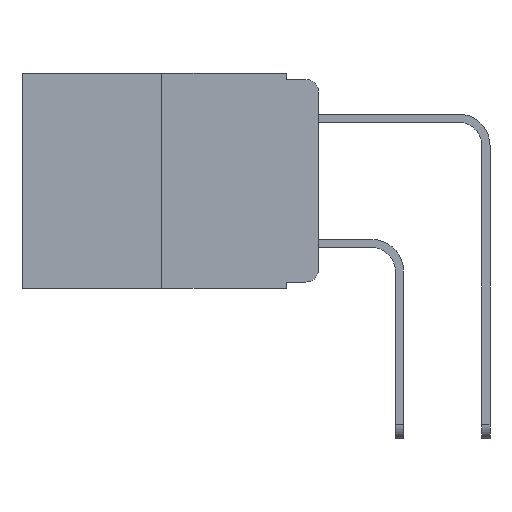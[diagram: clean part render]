
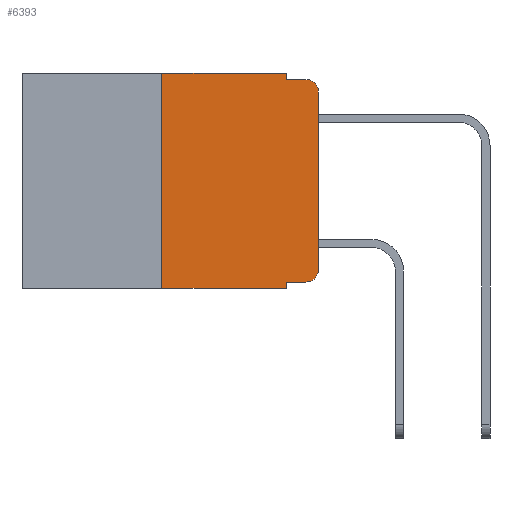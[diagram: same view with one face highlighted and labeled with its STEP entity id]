
A CAD part, left-side view. The second image highlights one B-rep face of the part: STEP entity #6393.
In plain terms, the highlighted planar face has unit normal (-1, 0, 0).
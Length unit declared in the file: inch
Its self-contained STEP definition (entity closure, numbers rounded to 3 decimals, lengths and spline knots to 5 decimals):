
#328 = ORIENTED_EDGE ( 'NONE', *, *, #4727, .F. ) ;
#359 = CIRCLE ( 'NONE', #1858, 0.02 ) ;
#385 = DIRECTION ( 'NONE',  ( -1., 0., 0. ) ) ;
#634 = ORIENTED_EDGE ( 'NONE', *, *, #3412, .T. ) ;
#791 = ORIENTED_EDGE ( 'NONE', *, *, #3538, .F. ) ;
#983 = VECTOR ( 'NONE', #6883, 39.37008 ) ;
#1095 = ORIENTED_EDGE ( 'NONE', *, *, #1416, .T. ) ;
#1416 = EDGE_CURVE ( 'NONE', #10333, #5225, #6491, .T. ) ;
#1601 = VECTOR ( 'NONE', #13738, 39.37008 ) ;
#1858 = AXIS2_PLACEMENT_3D ( 'NONE', #7493, #385, #8627 ) ;
#2063 = CARTESIAN_POINT ( 'NONE',  ( 0., 0.473, 0. ) ) ;
#2065 = PLANE ( 'NONE',  #14643 ) ;
#2159 = CIRCLE ( 'NONE', #10246, 0.02 ) ;
#2265 = ORIENTED_EDGE ( 'NONE', *, *, #6985, .T. ) ;
#2274 = EDGE_CURVE ( 'NONE', #12450, #3481, #10789, .T. ) ;
#2370 = CARTESIAN_POINT ( 'NONE',  ( 0., 0., -0.313 ) ) ;
#2591 = CARTESIAN_POINT ( 'NONE',  ( 0., 0.051, -0.333 ) ) ;
#2628 = ORIENTED_EDGE ( 'NONE', *, *, #2274, .F. ) ;
#2881 = CARTESIAN_POINT ( 'NONE',  ( 0., 0., 0. ) ) ;
#3010 = VECTOR ( 'NONE', #8505, 39.37008 ) ;
#3142 = VECTOR ( 'NONE', #12674, 39.37008 ) ;
#3370 = VERTEX_POINT ( 'NONE', #8922 ) ;
#3405 = DIRECTION ( 'NONE',  ( 0., 0., -1. ) ) ;
#3412 = EDGE_CURVE ( 'NONE', #5357, #10333, #2159, .T. ) ;
#3481 = VERTEX_POINT ( 'NONE', #6370 ) ;
#3538 = EDGE_CURVE ( 'NONE', #3481, #3671, #9909, .T. ) ;
#3671 = VERTEX_POINT ( 'NONE', #13999 ) ;
#3916 = EDGE_CURVE ( 'NONE', #3671, #13703, #9902, .T. ) ;
#4099 = DIRECTION ( 'NONE',  ( 0., -1., 0. ) ) ;
#4421 = EDGE_LOOP ( 'NONE', ( #1095, #2265, #328, #5591, #791, #2628, #11192, #5495, #7170, #634 ) ) ;
#4689 = DIRECTION ( 'NONE',  ( 0., 0., -1. ) ) ;
#4707 = DIRECTION ( 'NONE',  ( 1., 0., 0. ) ) ;
#4727 = EDGE_CURVE ( 'NONE', #13703, #3370, #6270, .T. ) ;
#4757 = VERTEX_POINT ( 'NONE', #12067 ) ;
#5158 = VECTOR ( 'NONE', #4099, 39.37008 ) ;
#5159 = CARTESIAN_POINT ( 'NONE',  ( 0., 0.473, 0. ) ) ;
#5225 = VERTEX_POINT ( 'NONE', #14273 ) ;
#5357 = VERTEX_POINT ( 'NONE', #7794 ) ;
#5495 = ORIENTED_EDGE ( 'NONE', *, *, #7742, .F. ) ;
#5583 = LINE ( 'NONE', #2591, #13869 ) ;
#5591 = ORIENTED_EDGE ( 'NONE', *, *, #3916, .F. ) ;
#6252 = DIRECTION ( 'NONE',  ( 0., 0., -1. ) ) ;
#6270 = LINE ( 'NONE', #11668, #3142 ) ;
#6271 = DIRECTION ( 'NONE',  ( 0., -1., 0. ) ) ;
#6336 = EDGE_CURVE ( 'NONE', #12450, #4757, #8492, .T. ) ;
#6370 = CARTESIAN_POINT ( 'NONE',  ( 0., 0.25, 0. ) ) ;
#6393 = ADVANCED_FACE ( 'NONE', ( #13505 ), #2065, .F. ) ;
#6491 = LINE ( 'NONE', #2881, #3010 ) ;
#6554 = CARTESIAN_POINT ( 'NONE',  ( 0., 0.25, -0.343 ) ) ;
#6874 = CARTESIAN_POINT ( 'NONE',  ( 0., 0.051, -0.333 ) ) ;
#6883 = DIRECTION ( 'NONE',  ( 0., 0., -1. ) ) ;
#6985 = EDGE_CURVE ( 'NONE', #5225, #3370, #359, .T. ) ;
#7009 = CARTESIAN_POINT ( 'NONE',  ( 0., 0.051, 0. ) ) ;
#7170 = ORIENTED_EDGE ( 'NONE', *, *, #9983, .T. ) ;
#7493 = CARTESIAN_POINT ( 'NONE',  ( 0., 0.02, -0.03 ) ) ;
#7742 = EDGE_CURVE ( 'NONE', #10996, #4757, #10012, .T. ) ;
#7794 = CARTESIAN_POINT ( 'NONE',  ( 0., 0.02, -0.333 ) ) ;
#8417 = DIRECTION ( 'NONE',  ( 0., -1., 0. ) ) ;
#8492 = LINE ( 'NONE', #13337, #5158 ) ;
#8505 = DIRECTION ( 'NONE',  ( 0., 0., 1. ) ) ;
#8627 = DIRECTION ( 'NONE',  ( 0., 0., -1. ) ) ;
#8922 = CARTESIAN_POINT ( 'NONE',  ( 0., 0.02, -0.01 ) ) ;
#9902 = LINE ( 'NONE', #7009, #983 ) ;
#9909 = LINE ( 'NONE', #5159, #12722 ) ;
#9983 = EDGE_CURVE ( 'NONE', #10996, #5357, #5583, .T. ) ;
#10012 = LINE ( 'NONE', #14340, #13465 ) ;
#10246 = AXIS2_PLACEMENT_3D ( 'NONE', #11680, #10644, #6252 ) ;
#10333 = VERTEX_POINT ( 'NONE', #2370 ) ;
#10466 = CARTESIAN_POINT ( 'NONE',  ( 0., 0.25, 0. ) ) ;
#10644 = DIRECTION ( 'NONE',  ( -1., 0., 0. ) ) ;
#10789 = LINE ( 'NONE', #10466, #1601 ) ;
#10996 = VERTEX_POINT ( 'NONE', #6874 ) ;
#11192 = ORIENTED_EDGE ( 'NONE', *, *, #6336, .T. ) ;
#11337 = CARTESIAN_POINT ( 'NONE',  ( 0., 0.051, -0.01 ) ) ;
#11668 = CARTESIAN_POINT ( 'NONE',  ( 0., 0.051, -0.01 ) ) ;
#11680 = CARTESIAN_POINT ( 'NONE',  ( 0., 0.02, -0.313 ) ) ;
#12067 = CARTESIAN_POINT ( 'NONE',  ( 0., 0.051, -0.343 ) ) ;
#12450 = VERTEX_POINT ( 'NONE', #6554 ) ;
#12674 = DIRECTION ( 'NONE',  ( 0., -1., 0. ) ) ;
#12722 = VECTOR ( 'NONE', #6271, 39.37008 ) ;
#13337 = CARTESIAN_POINT ( 'NONE',  ( 0., 0.473, -0.343 ) ) ;
#13465 = VECTOR ( 'NONE', #3405, 39.37008 ) ;
#13505 = FACE_OUTER_BOUND ( 'NONE', #4421, .T. ) ;
#13703 = VERTEX_POINT ( 'NONE', #11337 ) ;
#13738 = DIRECTION ( 'NONE',  ( 0., 0., 1. ) ) ;
#13869 = VECTOR ( 'NONE', #8417, 39.37008 ) ;
#13999 = CARTESIAN_POINT ( 'NONE',  ( 0., 0.051, 0. ) ) ;
#14273 = CARTESIAN_POINT ( 'NONE',  ( 0., 0., -0.03 ) ) ;
#14340 = CARTESIAN_POINT ( 'NONE',  ( 0., 0.051, 0. ) ) ;
#14643 = AXIS2_PLACEMENT_3D ( 'NONE', #2063, #4707, #4689 ) ;
